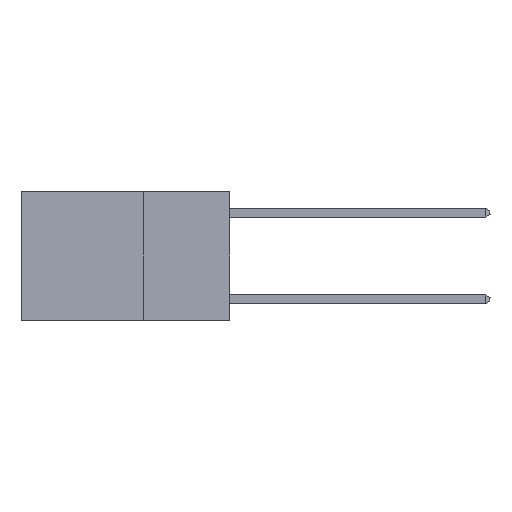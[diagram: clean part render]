
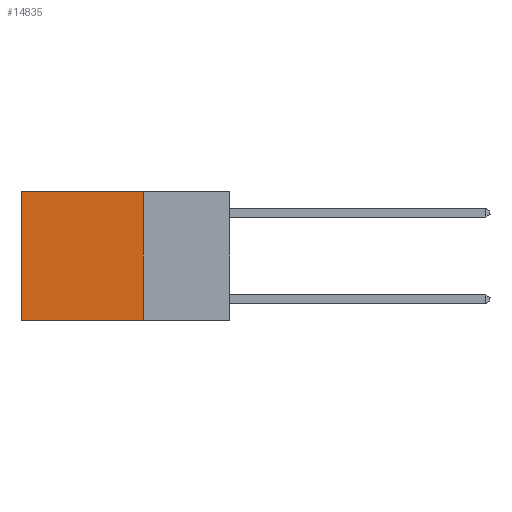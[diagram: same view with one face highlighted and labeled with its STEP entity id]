
A CAD part, left-side view. The second image highlights one B-rep face of the part: STEP entity #14835.
In plain terms, the highlighted planar face has unit normal (-1, 0, 0).
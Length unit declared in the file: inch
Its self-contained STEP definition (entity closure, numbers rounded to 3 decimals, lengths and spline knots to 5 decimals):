
#792 = CARTESIAN_POINT ( 'NONE',  ( 0.2625, 0.25, -0.37 ) ) ;
#1317 = AXIS2_PLACEMENT_3D ( 'NONE', #3734, #12561, #19743 ) ;
#1851 = LINE ( 'NONE', #14552, #10962 ) ;
#1957 = DIRECTION ( 'NONE',  ( 0., 1., 0. ) ) ;
#3699 = VECTOR ( 'NONE', #5775, 39.37008 ) ;
#3734 = CARTESIAN_POINT ( 'NONE',  ( 0.2625, 0.25, 0. ) ) ;
#3897 = LINE ( 'NONE', #19920, #3699 ) ;
#5775 = DIRECTION ( 'NONE',  ( 0., 1., 0. ) ) ;
#5952 = LINE ( 'NONE', #6067, #7420 ) ;
#6067 = CARTESIAN_POINT ( 'NONE',  ( 0.2625, 0.6, 0. ) ) ;
#6115 = LINE ( 'NONE', #13304, #18474 ) ;
#6911 = EDGE_CURVE ( 'NONE', #12394, #18901, #5952, .T. ) ;
#6926 = VERTEX_POINT ( 'NONE', #792 ) ;
#7420 = VECTOR ( 'NONE', #18776, 39.37008 ) ;
#7602 = ORIENTED_EDGE ( 'NONE', *, *, #21091, .F. ) ;
#8641 = CARTESIAN_POINT ( 'NONE',  ( 0.2625, 0.6, 0. ) ) ;
#10415 = CARTESIAN_POINT ( 'NONE',  ( 0.2625, 0.25, 0. ) ) ;
#10581 = EDGE_CURVE ( 'NONE', #18613, #12394, #1851, .T. ) ;
#10962 = VECTOR ( 'NONE', #1957, 39.37008 ) ;
#12394 = VERTEX_POINT ( 'NONE', #8641 ) ;
#12561 = DIRECTION ( 'NONE',  ( 1., 0., 0. ) ) ;
#12713 = EDGE_CURVE ( 'NONE', #18613, #6926, #6115, .T. ) ;
#13304 = CARTESIAN_POINT ( 'NONE',  ( 0.2625, 0.25, 0. ) ) ;
#14552 = CARTESIAN_POINT ( 'NONE',  ( 0.2625, 0.25, 0. ) ) ;
#14835 = ADVANCED_FACE ( 'NONE', ( #19863 ), #16101, .F. ) ;
#16101 = PLANE ( 'NONE',  #1317 ) ;
#16748 = CARTESIAN_POINT ( 'NONE',  ( 0.2625, 0.6, -0.37 ) ) ;
#16986 = EDGE_LOOP ( 'NONE', ( #19753, #7602, #18734, #21172 ) ) ;
#18474 = VECTOR ( 'NONE', #20491, 39.37008 ) ;
#18613 = VERTEX_POINT ( 'NONE', #10415 ) ;
#18734 = ORIENTED_EDGE ( 'NONE', *, *, #12713, .F. ) ;
#18776 = DIRECTION ( 'NONE',  ( 0., 0., -1. ) ) ;
#18901 = VERTEX_POINT ( 'NONE', #16748 ) ;
#19743 = DIRECTION ( 'NONE',  ( 0., 0., -1. ) ) ;
#19753 = ORIENTED_EDGE ( 'NONE', *, *, #6911, .T. ) ;
#19863 = FACE_OUTER_BOUND ( 'NONE', #16986, .T. ) ;
#19920 = CARTESIAN_POINT ( 'NONE',  ( 0.2625, 0.25, -0.37 ) ) ;
#20491 = DIRECTION ( 'NONE',  ( 0., 0., -1. ) ) ;
#21091 = EDGE_CURVE ( 'NONE', #6926, #18901, #3897, .T. ) ;
#21172 = ORIENTED_EDGE ( 'NONE', *, *, #10581, .T. ) ;
